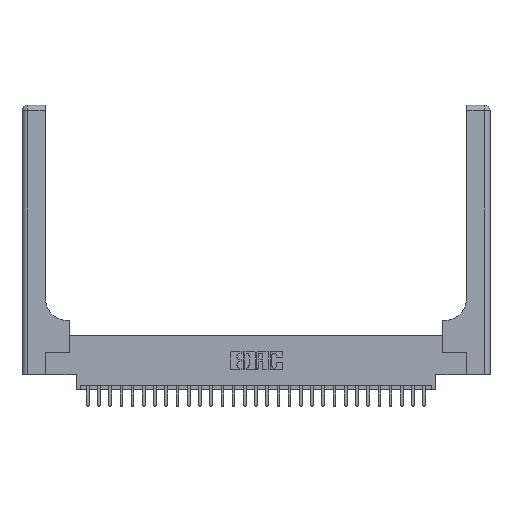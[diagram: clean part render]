
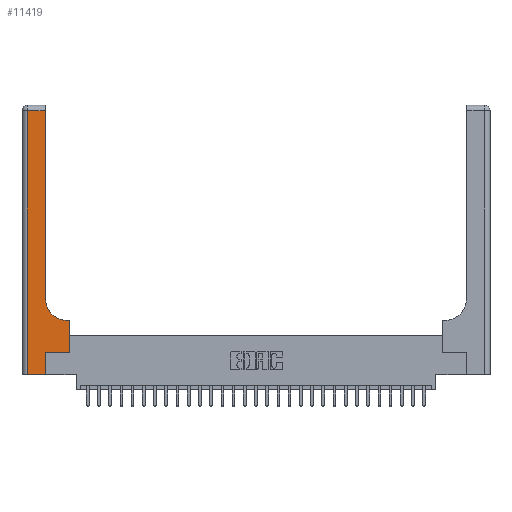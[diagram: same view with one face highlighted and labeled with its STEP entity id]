
A CAD part, top view. The second image highlights one B-rep face of the part: STEP entity #11419.
In plain terms, the highlighted planar face has unit normal (0, 0, 1).
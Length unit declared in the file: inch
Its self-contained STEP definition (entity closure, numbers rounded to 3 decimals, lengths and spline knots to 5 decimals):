
#4 = LINE ( 'NONE', #282, #1388 ) ;
#124 = VERTEX_POINT ( 'NONE', #23827 ) ;
#141 = DIRECTION ( 'NONE',  ( 0., 1., 0. ) ) ;
#282 = CARTESIAN_POINT ( 'NONE',  ( 0.528, 0.25, 0.37 ) ) ;
#1388 = VECTOR ( 'NONE', #141, 39.37008 ) ;
#1416 = ORIENTED_EDGE ( 'NONE', *, *, #21419, .T. ) ;
#1492 = ORIENTED_EDGE ( 'NONE', *, *, #11313, .T. ) ;
#1561 = ORIENTED_EDGE ( 'NONE', *, *, #18337, .T. ) ;
#2190 = LINE ( 'NONE', #4574, #13029 ) ;
#2916 = ORIENTED_EDGE ( 'NONE', *, *, #13059, .T. ) ;
#3711 = LINE ( 'NONE', #27588, #4262 ) ;
#3932 = AXIS2_PLACEMENT_3D ( 'NONE', #25395, #10057, #27073 ) ;
#4088 = CARTESIAN_POINT ( 'NONE',  ( 0.06, 3., 0.37 ) ) ;
#4262 = VECTOR ( 'NONE', #25475, 39.37008 ) ;
#4574 = CARTESIAN_POINT ( 'NONE',  ( 0., 0., 0.37 ) ) ;
#4698 = EDGE_CURVE ( 'NONE', #16089, #23647, #4, .T. ) ;
#5532 = ORIENTED_EDGE ( 'NONE', *, *, #18763, .T. ) ;
#6418 = CARTESIAN_POINT ( 'NONE',  ( 0.26, 2.94, 0.37 ) ) ;
#6530 = VERTEX_POINT ( 'NONE', #6418 ) ;
#7018 = VERTEX_POINT ( 'NONE', #24829 ) ;
#8637 = CARTESIAN_POINT ( 'NONE',  ( 0.51, 0.6, 0.37 ) ) ;
#10057 = DIRECTION ( 'NONE',  ( 0., 0., -1. ) ) ;
#10443 = CARTESIAN_POINT ( 'NONE',  ( 0.265, 0., 0.37 ) ) ;
#10756 = CARTESIAN_POINT ( 'NONE',  ( 0.265, 0.25, 0.37 ) ) ;
#10984 = AXIS2_PLACEMENT_3D ( 'NONE', #26784, #17986, #17849 ) ;
#11104 = CARTESIAN_POINT ( 'NONE',  ( 0.26, 3., 0.37 ) ) ;
#11261 = ORIENTED_EDGE ( 'NONE', *, *, #4698, .T. ) ;
#11313 = EDGE_CURVE ( 'NONE', #12170, #16089, #21481, .T. ) ;
#11419 = ADVANCED_FACE ( 'NONE', ( #13398 ), #26381, .F. ) ;
#11908 = EDGE_LOOP ( 'NONE', ( #5532, #1561, #1416, #15178, #13451, #1492, #11261, #15157, #2916 ) ) ;
#12170 = VERTEX_POINT ( 'NONE', #19289 ) ;
#12296 = VECTOR ( 'NONE', #19597, 39.37008 ) ;
#12383 = LINE ( 'NONE', #10443, #27092 ) ;
#13029 = VECTOR ( 'NONE', #15441, 39.37008 ) ;
#13059 = EDGE_CURVE ( 'NONE', #13107, #124, #22182, .T. ) ;
#13107 = VERTEX_POINT ( 'NONE', #8637 ) ;
#13398 = FACE_OUTER_BOUND ( 'NONE', #11908, .T. ) ;
#13451 = ORIENTED_EDGE ( 'NONE', *, *, #15783, .T. ) ;
#13630 = DIRECTION ( 'NONE',  ( -1., 0., 0. ) ) ;
#13706 = VECTOR ( 'NONE', #25852, 39.37008 ) ;
#13760 = CARTESIAN_POINT ( 'NONE',  ( 0., 2.94, 0.37 ) ) ;
#15157 = ORIENTED_EDGE ( 'NONE', *, *, #18552, .T. ) ;
#15178 = ORIENTED_EDGE ( 'NONE', *, *, #17118, .T. ) ;
#15230 = LINE ( 'NONE', #4088, #13706 ) ;
#15441 = DIRECTION ( 'NONE',  ( 1., 0., 0. ) ) ;
#15569 = CARTESIAN_POINT ( 'NONE',  ( 0.528, 0.25, 0.37 ) ) ;
#15783 = EDGE_CURVE ( 'NONE', #20066, #12170, #12383, .T. ) ;
#15985 = VERTEX_POINT ( 'NONE', #23400 ) ;
#16089 = VERTEX_POINT ( 'NONE', #15569 ) ;
#17118 = EDGE_CURVE ( 'NONE', #15985, #20066, #2190, .T. ) ;
#17849 = DIRECTION ( 'NONE',  ( -1., 0., 0. ) ) ;
#17915 = CARTESIAN_POINT ( 'NONE',  ( 0.528, 0.6, 0.37 ) ) ;
#17986 = DIRECTION ( 'NONE',  ( 0., 0., -1. ) ) ;
#18337 = EDGE_CURVE ( 'NONE', #6530, #7018, #20167, .T. ) ;
#18513 = DIRECTION ( 'NONE',  ( 0., 1., 0. ) ) ;
#18552 = EDGE_CURVE ( 'NONE', #23647, #13107, #3711, .T. ) ;
#18763 = EDGE_CURVE ( 'NONE', #124, #6530, #26174, .T. ) ;
#19289 = CARTESIAN_POINT ( 'NONE',  ( 0.265, 0.25, 0.37 ) ) ;
#19597 = DIRECTION ( 'NONE',  ( 0., 1., 0. ) ) ;
#20066 = VERTEX_POINT ( 'NONE', #24881 ) ;
#20167 = LINE ( 'NONE', #13760, #24714 ) ;
#21419 = EDGE_CURVE ( 'NONE', #7018, #15985, #15230, .T. ) ;
#21481 = LINE ( 'NONE', #10756, #27471 ) ;
#22182 = CIRCLE ( 'NONE', #3932, 0.25 ) ;
#23400 = CARTESIAN_POINT ( 'NONE',  ( 0.06, 0., 0.37 ) ) ;
#23456 = DIRECTION ( 'NONE',  ( 1., 0., 0. ) ) ;
#23647 = VERTEX_POINT ( 'NONE', #17915 ) ;
#23827 = CARTESIAN_POINT ( 'NONE',  ( 0.26, 0.85, 0.37 ) ) ;
#24714 = VECTOR ( 'NONE', #13630, 39.37008 ) ;
#24829 = CARTESIAN_POINT ( 'NONE',  ( 0.06, 2.94, 0.37 ) ) ;
#24881 = CARTESIAN_POINT ( 'NONE',  ( 0.265, 0., 0.37 ) ) ;
#25395 = CARTESIAN_POINT ( 'NONE',  ( 0.51, 0.85, 0.37 ) ) ;
#25475 = DIRECTION ( 'NONE',  ( -1., 0., 0. ) ) ;
#25852 = DIRECTION ( 'NONE',  ( 0., -1., 0. ) ) ;
#26174 = LINE ( 'NONE', #11104, #12296 ) ;
#26381 = PLANE ( 'NONE',  #10984 ) ;
#26784 = CARTESIAN_POINT ( 'NONE',  ( 0., 3., 0.37 ) ) ;
#27073 = DIRECTION ( 'NONE',  ( 1., 0., 0. ) ) ;
#27092 = VECTOR ( 'NONE', #18513, 39.37008 ) ;
#27471 = VECTOR ( 'NONE', #23456, 39.37008 ) ;
#27588 = CARTESIAN_POINT ( 'NONE',  ( 0.26, 0.6, 0.37 ) ) ;
